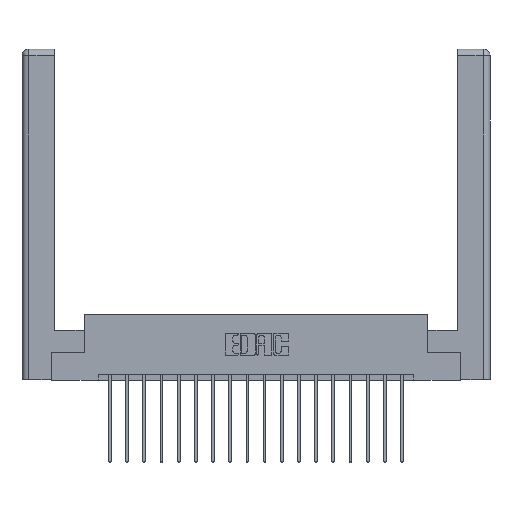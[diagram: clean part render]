
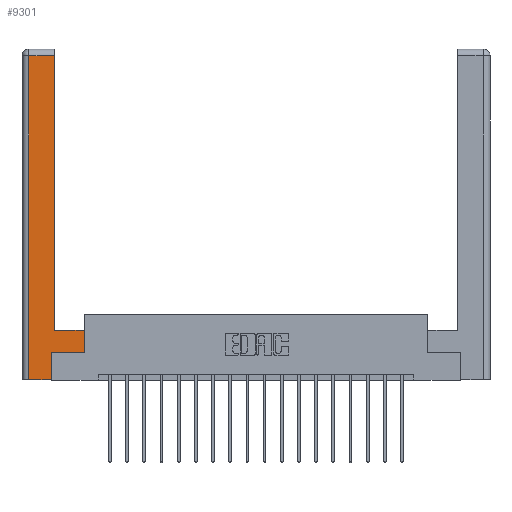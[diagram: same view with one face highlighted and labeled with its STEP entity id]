
A CAD part, top view. The second image highlights one B-rep face of the part: STEP entity #9301.
In plain terms, the highlighted planar face has unit normal (0, 0, 1).
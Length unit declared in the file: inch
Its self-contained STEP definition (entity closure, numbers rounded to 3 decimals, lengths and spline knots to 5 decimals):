
#125 = VECTOR ( 'NONE', #15077, 39.37008 ) ;
#812 = DIRECTION ( 'NONE',  ( 0., -1., 0. ) ) ;
#933 = CARTESIAN_POINT ( 'NONE',  ( 0.0615, 0., 0. ) ) ;
#1193 = VERTEX_POINT ( 'NONE', #9680 ) ;
#1321 = VERTEX_POINT ( 'NONE', #5255 ) ;
#1959 = VECTOR ( 'NONE', #9966, 39.37008 ) ;
#2508 = ORIENTED_EDGE ( 'NONE', *, *, #7227, .T. ) ;
#2820 = EDGE_CURVE ( 'NONE', #19007, #17127, #10402, .T. ) ;
#3186 = EDGE_CURVE ( 'NONE', #1321, #8367, #17290, .T. ) ;
#4105 = ORIENTED_EDGE ( 'NONE', *, *, #5186, .T. ) ;
#4401 = ORIENTED_EDGE ( 'NONE', *, *, #16635, .T. ) ;
#4412 = CARTESIAN_POINT ( 'NONE',  ( 0., 0., 0. ) ) ;
#4464 = DIRECTION ( 'NONE',  ( -1., 0., 0. ) ) ;
#4683 = DIRECTION ( 'NONE',  ( 0., 1., 0. ) ) ;
#4696 = CARTESIAN_POINT ( 'NONE',  ( 0.0615, 0., 0. ) ) ;
#4715 = VECTOR ( 'NONE', #812, 39.37008 ) ;
#4783 = CARTESIAN_POINT ( 'NONE',  ( 0.565, 0.245, 0. ) ) ;
#5160 = VECTOR ( 'NONE', #9186, 39.37008 ) ;
#5186 = EDGE_CURVE ( 'NONE', #8367, #14328, #8173, .T. ) ;
#5255 = CARTESIAN_POINT ( 'NONE',  ( 0.265, 0., 0. ) ) ;
#5360 = EDGE_CURVE ( 'NONE', #18917, #1193, #9356, .T. ) ;
#5727 = CARTESIAN_POINT ( 'NONE',  ( 0.0615, 2.94, 0. ) ) ;
#6629 = CARTESIAN_POINT ( 'NONE',  ( 0.295, 0.45, 0. ) ) ;
#7147 = FACE_OUTER_BOUND ( 'NONE', #16130, .T. ) ;
#7227 = EDGE_CURVE ( 'NONE', #8948, #1321, #12677, .T. ) ;
#8173 = LINE ( 'NONE', #15901, #1959 ) ;
#8367 = VERTEX_POINT ( 'NONE', #17659 ) ;
#8948 = VERTEX_POINT ( 'NONE', #4696 ) ;
#9186 = DIRECTION ( 'NONE',  ( 0., 1., 0. ) ) ;
#9193 = DIRECTION ( 'NONE',  ( -1., 0., 0. ) ) ;
#9301 = ADVANCED_FACE ( 'NONE', ( #7147 ), #15936, .F. ) ;
#9356 = LINE ( 'NONE', #5727, #9843 ) ;
#9680 = CARTESIAN_POINT ( 'NONE',  ( 0.0615, 2.94, 0. ) ) ;
#9843 = VECTOR ( 'NONE', #4464, 39.37008 ) ;
#9966 = DIRECTION ( 'NONE',  ( 1., 0., 0. ) ) ;
#10402 = LINE ( 'NONE', #13762, #15385 ) ;
#10427 = CARTESIAN_POINT ( 'NONE',  ( 0.295, 3., 0. ) ) ;
#10613 = ORIENTED_EDGE ( 'NONE', *, *, #2820, .T. ) ;
#10729 = EDGE_CURVE ( 'NONE', #1193, #8948, #13983, .T. ) ;
#10869 = DIRECTION ( 'NONE',  ( 1., 0., 0. ) ) ;
#11519 = CARTESIAN_POINT ( 'NONE',  ( 0.265, 0.245, 0. ) ) ;
#12126 = CARTESIAN_POINT ( 'NONE',  ( 0.265, 0., 0. ) ) ;
#12457 = VECTOR ( 'NONE', #10869, 39.37008 ) ;
#12677 = LINE ( 'NONE', #12126, #12457 ) ;
#13551 = ORIENTED_EDGE ( 'NONE', *, *, #3186, .T. ) ;
#13731 = CARTESIAN_POINT ( 'NONE',  ( 0.295, 2.94, 0. ) ) ;
#13762 = CARTESIAN_POINT ( 'NONE',  ( 0.295, 0.45, 0. ) ) ;
#13983 = LINE ( 'NONE', #933, #4715 ) ;
#14222 = LINE ( 'NONE', #18575, #17058 ) ;
#14328 = VERTEX_POINT ( 'NONE', #4783 ) ;
#15077 = DIRECTION ( 'NONE',  ( 0., 1., 0. ) ) ;
#15125 = CARTESIAN_POINT ( 'NONE',  ( 0.565, 0.45, 0. ) ) ;
#15385 = VECTOR ( 'NONE', #9193, 39.37008 ) ;
#15416 = DIRECTION ( 'NONE',  ( 0., 0., -1. ) ) ;
#15604 = LINE ( 'NONE', #10427, #125 ) ;
#15901 = CARTESIAN_POINT ( 'NONE',  ( 0.565, 0.245, 0. ) ) ;
#15936 = PLANE ( 'NONE',  #18692 ) ;
#16130 = EDGE_LOOP ( 'NONE', ( #4401, #19079, #17980, #2508, #13551, #4105, #17119, #10613 ) ) ;
#16635 = EDGE_CURVE ( 'NONE', #17127, #18917, #15604, .T. ) ;
#17058 = VECTOR ( 'NONE', #4683, 39.37008 ) ;
#17086 = DIRECTION ( 'NONE',  ( -1., 0., 0. ) ) ;
#17119 = ORIENTED_EDGE ( 'NONE', *, *, #19051, .T. ) ;
#17127 = VERTEX_POINT ( 'NONE', #6629 ) ;
#17290 = LINE ( 'NONE', #11519, #5160 ) ;
#17659 = CARTESIAN_POINT ( 'NONE',  ( 0.265, 0.245, 0. ) ) ;
#17980 = ORIENTED_EDGE ( 'NONE', *, *, #10729, .T. ) ;
#18575 = CARTESIAN_POINT ( 'NONE',  ( 0.565, 0.45, 0. ) ) ;
#18692 = AXIS2_PLACEMENT_3D ( 'NONE', #4412, #15416, #17086 ) ;
#18917 = VERTEX_POINT ( 'NONE', #13731 ) ;
#19007 = VERTEX_POINT ( 'NONE', #15125 ) ;
#19051 = EDGE_CURVE ( 'NONE', #14328, #19007, #14222, .T. ) ;
#19079 = ORIENTED_EDGE ( 'NONE', *, *, #5360, .T. ) ;
